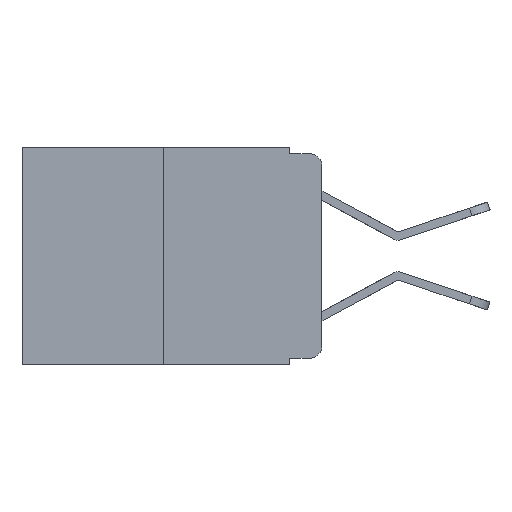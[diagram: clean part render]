
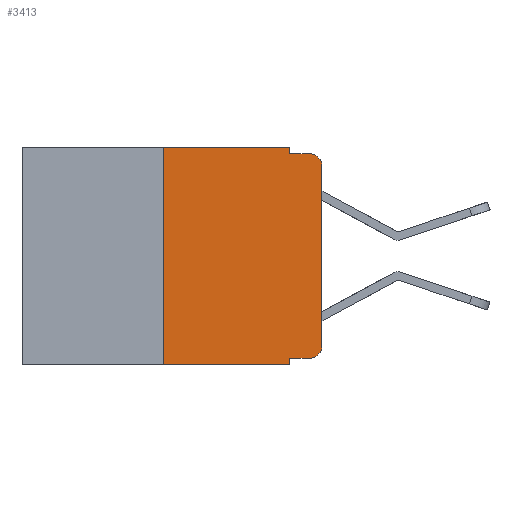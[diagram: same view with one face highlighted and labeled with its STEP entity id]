
A CAD part, left-side view. The second image highlights one B-rep face of the part: STEP entity #3413.
In plain terms, the highlighted planar face has unit normal (-1, 0, 0).
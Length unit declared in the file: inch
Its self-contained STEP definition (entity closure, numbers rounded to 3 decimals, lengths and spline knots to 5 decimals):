
#52 = ORIENTED_EDGE ( 'NONE', *, *, #10431, .T. ) ;
#55 = LINE ( 'NONE', #8577, #4938 ) ;
#69 = CARTESIAN_POINT ( 'NONE',  ( 0., 0., -0.313 ) ) ;
#197 = DIRECTION ( 'NONE',  ( 0., 0., 1. ) ) ;
#208 = ORIENTED_EDGE ( 'NONE', *, *, #4262, .T. ) ;
#314 = DIRECTION ( 'NONE',  ( 0., -1., 0. ) ) ;
#499 = CARTESIAN_POINT ( 'NONE',  ( 0., 0.25, 0. ) ) ;
#805 = VECTOR ( 'NONE', #8776, 39.37008 ) ;
#1206 = EDGE_CURVE ( 'NONE', #8141, #5279, #2883, .T. ) ;
#1278 = CARTESIAN_POINT ( 'NONE',  ( 0., 0.02, -0.03 ) ) ;
#1283 = VERTEX_POINT ( 'NONE', #8179 ) ;
#1725 = VECTOR ( 'NONE', #9600, 39.37008 ) ;
#1824 = VECTOR ( 'NONE', #314, 39.37008 ) ;
#1840 = CARTESIAN_POINT ( 'NONE',  ( 0., 0.051, 0. ) ) ;
#2091 = CIRCLE ( 'NONE', #3954, 0.02 ) ;
#2159 = AXIS2_PLACEMENT_3D ( 'NONE', #11332, #11287, #8853 ) ;
#2167 = DIRECTION ( 'NONE',  ( 0., 0., -1. ) ) ;
#2377 = CARTESIAN_POINT ( 'NONE',  ( 0., 0.25, 0. ) ) ;
#2428 = EDGE_CURVE ( 'NONE', #5279, #5849, #6664, .T. ) ;
#2607 = CARTESIAN_POINT ( 'NONE',  ( 0., 0.051, -0.01 ) ) ;
#2883 = LINE ( 'NONE', #1840, #8800 ) ;
#2933 = CARTESIAN_POINT ( 'NONE',  ( 0., 0., 0. ) ) ;
#2948 = EDGE_LOOP ( 'NONE', ( #5653, #208, #4177, #6691, #4173, #3956, #52, #3793, #4952, #3500 ) ) ;
#3174 = DIRECTION ( 'NONE',  ( 0., 0., -1. ) ) ;
#3285 = EDGE_CURVE ( 'NONE', #11042, #6649, #7515, .T. ) ;
#3413 = ADVANCED_FACE ( 'NONE', ( #3992 ), #6178, .F. ) ;
#3500 = ORIENTED_EDGE ( 'NONE', *, *, #3285, .T. ) ;
#3793 = ORIENTED_EDGE ( 'NONE', *, *, #8714, .F. ) ;
#3864 = CARTESIAN_POINT ( 'NONE',  ( 0., 0.473, 0. ) ) ;
#3930 = EDGE_CURVE ( 'NONE', #10441, #8141, #7922, .T. ) ;
#3954 = AXIS2_PLACEMENT_3D ( 'NONE', #1278, #7609, #2167 ) ;
#3956 = ORIENTED_EDGE ( 'NONE', *, *, #10481, .F. ) ;
#3992 = FACE_OUTER_BOUND ( 'NONE', #2948, .T. ) ;
#4173 = ORIENTED_EDGE ( 'NONE', *, *, #3930, .F. ) ;
#4177 = ORIENTED_EDGE ( 'NONE', *, *, #2428, .F. ) ;
#4249 = CARTESIAN_POINT ( 'NONE',  ( 0., 0.051, -0.333 ) ) ;
#4262 = EDGE_CURVE ( 'NONE', #6816, #5849, #2091, .T. ) ;
#4449 = LINE ( 'NONE', #2377, #1725 ) ;
#4926 = CARTESIAN_POINT ( 'NONE',  ( 0., 0.051, 0. ) ) ;
#4938 = VECTOR ( 'NONE', #3174, 39.37008 ) ;
#4952 = ORIENTED_EDGE ( 'NONE', *, *, #5141, .T. ) ;
#4970 = VECTOR ( 'NONE', #197, 39.37008 ) ;
#5024 = DIRECTION ( 'NONE',  ( 0., 0., -1. ) ) ;
#5052 = DIRECTION ( 'NONE',  ( 1., 0., 0. ) ) ;
#5053 = CARTESIAN_POINT ( 'NONE',  ( 0., 0.473, -0.343 ) ) ;
#5056 = LINE ( 'NONE', #5053, #7129 ) ;
#5141 = EDGE_CURVE ( 'NONE', #1283, #11042, #8031, .T. ) ;
#5279 = VERTEX_POINT ( 'NONE', #8965 ) ;
#5653 = ORIENTED_EDGE ( 'NONE', *, *, #6124, .T. ) ;
#5849 = VERTEX_POINT ( 'NONE', #9725 ) ;
#5951 = DIRECTION ( 'NONE',  ( 0., -1., 0. ) ) ;
#6124 = EDGE_CURVE ( 'NONE', #6649, #6816, #7334, .T. ) ;
#6178 = PLANE ( 'NONE',  #10046 ) ;
#6626 = CARTESIAN_POINT ( 'NONE',  ( 0., 0., -0.03 ) ) ;
#6638 = VERTEX_POINT ( 'NONE', #7297 ) ;
#6649 = VERTEX_POINT ( 'NONE', #69 ) ;
#6664 = LINE ( 'NONE', #2607, #1824 ) ;
#6691 = ORIENTED_EDGE ( 'NONE', *, *, #1206, .F. ) ;
#6816 = VERTEX_POINT ( 'NONE', #6626 ) ;
#7129 = VECTOR ( 'NONE', #9517, 39.37008 ) ;
#7297 = CARTESIAN_POINT ( 'NONE',  ( 0., 0.25, -0.343 ) ) ;
#7334 = LINE ( 'NONE', #2933, #4970 ) ;
#7407 = CARTESIAN_POINT ( 'NONE',  ( 0., 0.051, -0.343 ) ) ;
#7515 = CIRCLE ( 'NONE', #2159, 0.02 ) ;
#7609 = DIRECTION ( 'NONE',  ( -1., 0., 0. ) ) ;
#7636 = VECTOR ( 'NONE', #5951, 39.37008 ) ;
#7922 = LINE ( 'NONE', #3864, #7636 ) ;
#8005 = VERTEX_POINT ( 'NONE', #7407 ) ;
#8031 = LINE ( 'NONE', #4249, #805 ) ;
#8136 = CARTESIAN_POINT ( 'NONE',  ( 0., 0.473, 0. ) ) ;
#8141 = VERTEX_POINT ( 'NONE', #4926 ) ;
#8179 = CARTESIAN_POINT ( 'NONE',  ( 0., 0.051, -0.333 ) ) ;
#8477 = DIRECTION ( 'NONE',  ( 0., 0., -1. ) ) ;
#8577 = CARTESIAN_POINT ( 'NONE',  ( 0., 0.051, 0. ) ) ;
#8714 = EDGE_CURVE ( 'NONE', #1283, #8005, #55, .T. ) ;
#8776 = DIRECTION ( 'NONE',  ( 0., -1., 0. ) ) ;
#8800 = VECTOR ( 'NONE', #8477, 39.37008 ) ;
#8853 = DIRECTION ( 'NONE',  ( 0., 0., -1. ) ) ;
#8965 = CARTESIAN_POINT ( 'NONE',  ( 0., 0.051, -0.01 ) ) ;
#9517 = DIRECTION ( 'NONE',  ( 0., -1., 0. ) ) ;
#9600 = DIRECTION ( 'NONE',  ( 0., 0., 1. ) ) ;
#9725 = CARTESIAN_POINT ( 'NONE',  ( 0., 0.02, -0.01 ) ) ;
#10046 = AXIS2_PLACEMENT_3D ( 'NONE', #8136, #5052, #5024 ) ;
#10431 = EDGE_CURVE ( 'NONE', #6638, #8005, #5056, .T. ) ;
#10441 = VERTEX_POINT ( 'NONE', #499 ) ;
#10481 = EDGE_CURVE ( 'NONE', #6638, #10441, #4449, .T. ) ;
#11042 = VERTEX_POINT ( 'NONE', #11247 ) ;
#11247 = CARTESIAN_POINT ( 'NONE',  ( 0., 0.02, -0.333 ) ) ;
#11287 = DIRECTION ( 'NONE',  ( -1., 0., 0. ) ) ;
#11332 = CARTESIAN_POINT ( 'NONE',  ( 0., 0.02, -0.313 ) ) ;
